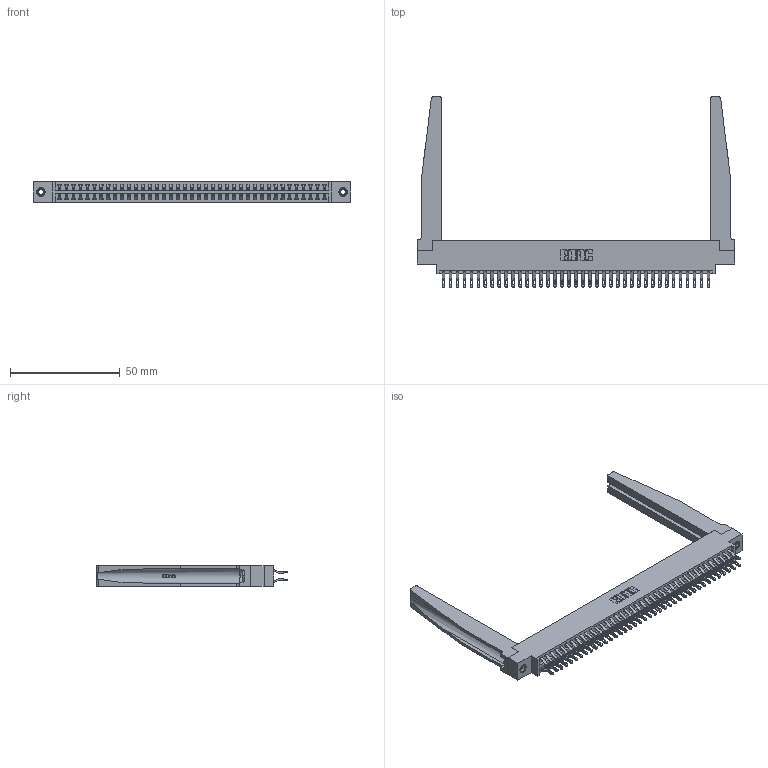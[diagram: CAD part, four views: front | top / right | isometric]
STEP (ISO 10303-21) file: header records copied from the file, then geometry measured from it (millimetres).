
FILE_DESCRIPTION (( 'STEP AP203' ), '1' );
FILE_NAME ('346-078-555-878.STEP', '2022-05-25T14:27:42', ( '' ), ( '' ), 'SwSTEP 2.0', 'SolidWorks 2020', '' );
FILE_SCHEMA (( 'CONFIG_CONTROL_DESIGN' ));
Length unit declared in the file: inch
Products named in the file (5): 345-292-001_555 Tail; 345-250-001_345-250-001-102; 346-078-555-878; 346-220-078_345-220-078; 346 Part_0.170 Offset - 0.156 Dia-TH
Assembly tree (83 placements, depth 2):
  346-078-555-878
    346 Part_0.170 Offset - 0.156 Dia-TH
    345-292-001_555 Tail  x78
    346-220-078_345-220-078  x2
    345-250-001_345-250-001-102  x2
Bounding box: 144.4 x 86.74 x 9.4 mm (x, y, z)
Volume: 21019.8 mm3; surface area: 26907.4 mm2
Topology: 83 solids, 83 shells, 4898 faces, 15259 edges, 10162 vertices
Faces by surface type: plane 2810, cylinder 2036, bspline 36, cone 12, torus 4
Entity records: 31478 total; most frequent: CARTESIAN_POINT 6171, ORIENTED_EDGE 4962, DIRECTION 4443, EDGE_CURVE 2481, VECTOR 2079, LINE 2079, VERTEX_POINT 1648, AXIS2_PLACEMENT_3D 1182
